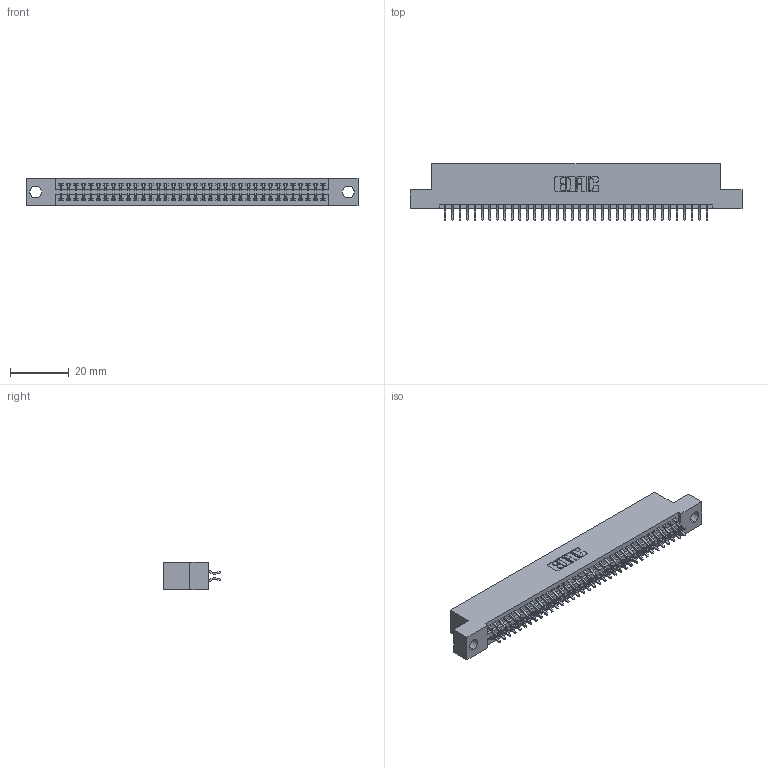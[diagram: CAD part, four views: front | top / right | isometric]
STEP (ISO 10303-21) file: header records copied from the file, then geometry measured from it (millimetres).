
FILE_DESCRIPTION (( 'STEP AP203' ), '1' );
FILE_NAME ('395-072-556-204.STEP', '2018-11-27T15:15:22', ( '' ), ( '' ), 'SwSTEP 2.0', 'SolidWorks 2016', '' );
FILE_SCHEMA (( 'CONFIG_CONTROL_DESIGN' ));
Length unit declared in the file: inch
Products named in the file (3): 345 Part_Flush Mounting Lugs - 0.156 Dia-TH; 345-292-001_556 Tail; 395-072-556-204
Assembly tree (73 placements, depth 2):
  395-072-556-204
    345 Part_Flush Mounting Lugs - 0.156 Dia-TH
    345-292-001_556 Tail  x72
Bounding box: 112.65 x 19.24 x 9.4 mm (x, y, z)
Volume: 10796.4 mm3; surface area: 15594.9 mm2
Topology: 73 solids, 73 shells, 4158 faces, 12365 edges, 8146 vertices
Faces by surface type: plane 2744, cylinder 1414
Entity records: 29277 total; most frequent: CARTESIAN_POINT 4928, ORIENTED_EDGE 4850, DIRECTION 4341, EDGE_CURVE 2425, LINE 2141, VECTOR 2141, VERTEX_POINT 1614, AXIS2_PLACEMENT_3D 1100
